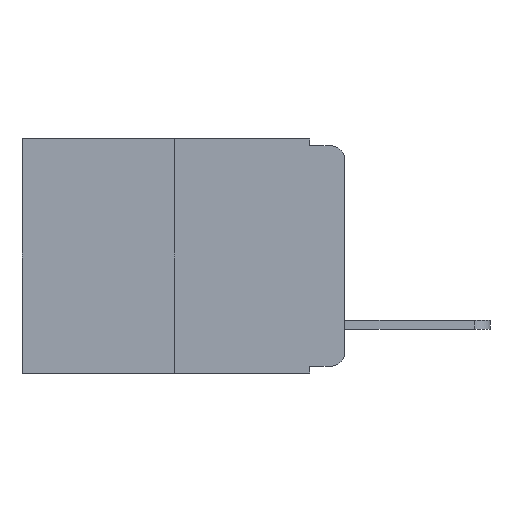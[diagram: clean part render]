
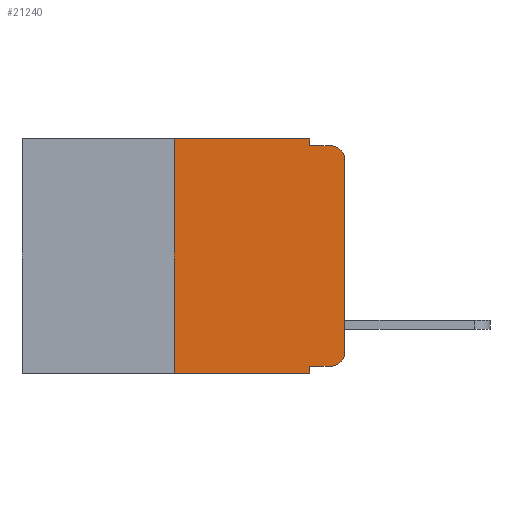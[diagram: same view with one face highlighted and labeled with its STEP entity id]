
A CAD part, left-side view. The second image highlights one B-rep face of the part: STEP entity #21240.
In plain terms, the highlighted planar face has unit normal (-1, 0, 0).
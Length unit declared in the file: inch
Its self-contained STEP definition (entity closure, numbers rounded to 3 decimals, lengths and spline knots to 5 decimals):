
#158 = LINE ( 'NONE', #11532, #16141 ) ;
#1208 = CARTESIAN_POINT ( 'NONE',  ( 0., 0., -0.313 ) ) ;
#1243 = CARTESIAN_POINT ( 'NONE',  ( 0., 0.051, 0. ) ) ;
#1330 = VERTEX_POINT ( 'NONE', #13670 ) ;
#1548 = DIRECTION ( 'NONE',  ( 0., 0., -1. ) ) ;
#1585 = VECTOR ( 'NONE', #7479, 39.37008 ) ;
#1831 = LINE ( 'NONE', #2767, #18935 ) ;
#2624 = LINE ( 'NONE', #8175, #14677 ) ;
#2767 = CARTESIAN_POINT ( 'NONE',  ( 0., 0.051, -0.333 ) ) ;
#3429 = VERTEX_POINT ( 'NONE', #8594 ) ;
#3885 = VERTEX_POINT ( 'NONE', #8642 ) ;
#4359 = AXIS2_PLACEMENT_3D ( 'NONE', #19349, #12285, #1548 ) ;
#4630 = CARTESIAN_POINT ( 'NONE',  ( 0., 0.25, 0. ) ) ;
#4822 = VECTOR ( 'NONE', #23052, 39.37008 ) ;
#4872 = EDGE_CURVE ( 'NONE', #3429, #10110, #1831, .T. ) ;
#4926 = LINE ( 'NONE', #16393, #1585 ) ;
#5212 = VERTEX_POINT ( 'NONE', #14293 ) ;
#5299 = VERTEX_POINT ( 'NONE', #19997 ) ;
#5352 = EDGE_CURVE ( 'NONE', #10110, #9798, #21223, .T. ) ;
#5466 = AXIS2_PLACEMENT_3D ( 'NONE', #13242, #13398, #17090 ) ;
#6333 = DIRECTION ( 'NONE',  ( 0., 0., 1. ) ) ;
#7089 = ORIENTED_EDGE ( 'NONE', *, *, #4872, .T. ) ;
#7340 = EDGE_CURVE ( 'NONE', #22330, #12878, #23071, .T. ) ;
#7479 = DIRECTION ( 'NONE',  ( 0., 0., 1. ) ) ;
#7715 = CARTESIAN_POINT ( 'NONE',  ( 0., 0.051, -0.01 ) ) ;
#8119 = EDGE_CURVE ( 'NONE', #3885, #8453, #18007, .T. ) ;
#8175 = CARTESIAN_POINT ( 'NONE',  ( 0., 0.051, 0. ) ) ;
#8344 = CARTESIAN_POINT ( 'NONE',  ( 0., 0.473, -0.343 ) ) ;
#8346 = CARTESIAN_POINT ( 'NONE',  ( 0., 0.02, -0.01 ) ) ;
#8396 = PLANE ( 'NONE',  #4359 ) ;
#8435 = VECTOR ( 'NONE', #22482, 39.37008 ) ;
#8453 = VERTEX_POINT ( 'NONE', #8346 ) ;
#8594 = CARTESIAN_POINT ( 'NONE',  ( 0., 0.051, -0.333 ) ) ;
#8642 = CARTESIAN_POINT ( 'NONE',  ( 0., 0., -0.03 ) ) ;
#8691 = VECTOR ( 'NONE', #19035, 39.37008 ) ;
#9508 = LINE ( 'NONE', #7715, #19366 ) ;
#9798 = VERTEX_POINT ( 'NONE', #1208 ) ;
#10110 = VERTEX_POINT ( 'NONE', #17916 ) ;
#10820 = EDGE_CURVE ( 'NONE', #1330, #5212, #22195, .T. ) ;
#11027 = ORIENTED_EDGE ( 'NONE', *, *, #14921, .F. ) ;
#11039 = ORIENTED_EDGE ( 'NONE', *, *, #8119, .T. ) ;
#11092 = ORIENTED_EDGE ( 'NONE', *, *, #5352, .T. ) ;
#11220 = LINE ( 'NONE', #1243, #8691 ) ;
#11532 = CARTESIAN_POINT ( 'NONE',  ( 0., 0.25, 0. ) ) ;
#11619 = ORIENTED_EDGE ( 'NONE', *, *, #18718, .F. ) ;
#12009 = DIRECTION ( 'NONE',  ( 0., 0., -1. ) ) ;
#12071 = EDGE_CURVE ( 'NONE', #12878, #5299, #2624, .T. ) ;
#12285 = DIRECTION ( 'NONE',  ( 1., 0., 0. ) ) ;
#12319 = ORIENTED_EDGE ( 'NONE', *, *, #7340, .F. ) ;
#12878 = VERTEX_POINT ( 'NONE', #21395 ) ;
#13162 = DIRECTION ( 'NONE',  ( 0., -1., 0. ) ) ;
#13182 = DIRECTION ( 'NONE',  ( 0., -1., 0. ) ) ;
#13242 = CARTESIAN_POINT ( 'NONE',  ( 0., 0.02, -0.313 ) ) ;
#13398 = DIRECTION ( 'NONE',  ( -1., 0., 0. ) ) ;
#13670 = CARTESIAN_POINT ( 'NONE',  ( 0., 0.25, -0.343 ) ) ;
#13705 = EDGE_CURVE ( 'NONE', #5299, #8453, #9508, .T. ) ;
#14141 = CARTESIAN_POINT ( 'NONE',  ( 0., 0.02, -0.03 ) ) ;
#14293 = CARTESIAN_POINT ( 'NONE',  ( 0., 0.051, -0.343 ) ) ;
#14677 = VECTOR ( 'NONE', #17649, 39.37008 ) ;
#14777 = FACE_OUTER_BOUND ( 'NONE', #16523, .T. ) ;
#14921 = EDGE_CURVE ( 'NONE', #3429, #5212, #11220, .T. ) ;
#15425 = AXIS2_PLACEMENT_3D ( 'NONE', #14141, #17758, #12009 ) ;
#16141 = VECTOR ( 'NONE', #6333, 39.37008 ) ;
#16393 = CARTESIAN_POINT ( 'NONE',  ( 0., 0., 0. ) ) ;
#16523 = EDGE_LOOP ( 'NONE', ( #18420, #11039, #19501, #22653, #12319, #11619, #22423, #11027, #7089, #11092 ) ) ;
#17090 = DIRECTION ( 'NONE',  ( 0., 0., -1. ) ) ;
#17649 = DIRECTION ( 'NONE',  ( 0., 0., -1. ) ) ;
#17758 = DIRECTION ( 'NONE',  ( -1., 0., 0. ) ) ;
#17916 = CARTESIAN_POINT ( 'NONE',  ( 0., 0.02, -0.333 ) ) ;
#18007 = CIRCLE ( 'NONE', #15425, 0.02 ) ;
#18420 = ORIENTED_EDGE ( 'NONE', *, *, #22613, .T. ) ;
#18718 = EDGE_CURVE ( 'NONE', #1330, #22330, #158, .T. ) ;
#18935 = VECTOR ( 'NONE', #13182, 39.37008 ) ;
#19035 = DIRECTION ( 'NONE',  ( 0., 0., -1. ) ) ;
#19349 = CARTESIAN_POINT ( 'NONE',  ( 0., 0.473, 0. ) ) ;
#19366 = VECTOR ( 'NONE', #13162, 39.37008 ) ;
#19501 = ORIENTED_EDGE ( 'NONE', *, *, #13705, .F. ) ;
#19602 = CARTESIAN_POINT ( 'NONE',  ( 0., 0.473, 0. ) ) ;
#19997 = CARTESIAN_POINT ( 'NONE',  ( 0., 0.051, -0.01 ) ) ;
#21223 = CIRCLE ( 'NONE', #5466, 0.02 ) ;
#21240 = ADVANCED_FACE ( 'NONE', ( #14777 ), #8396, .F. ) ;
#21395 = CARTESIAN_POINT ( 'NONE',  ( 0., 0.051, 0. ) ) ;
#22195 = LINE ( 'NONE', #8344, #8435 ) ;
#22330 = VERTEX_POINT ( 'NONE', #4630 ) ;
#22423 = ORIENTED_EDGE ( 'NONE', *, *, #10820, .T. ) ;
#22482 = DIRECTION ( 'NONE',  ( 0., -1., 0. ) ) ;
#22613 = EDGE_CURVE ( 'NONE', #9798, #3885, #4926, .T. ) ;
#22653 = ORIENTED_EDGE ( 'NONE', *, *, #12071, .F. ) ;
#23052 = DIRECTION ( 'NONE',  ( 0., -1., 0. ) ) ;
#23071 = LINE ( 'NONE', #19602, #4822 ) ;
